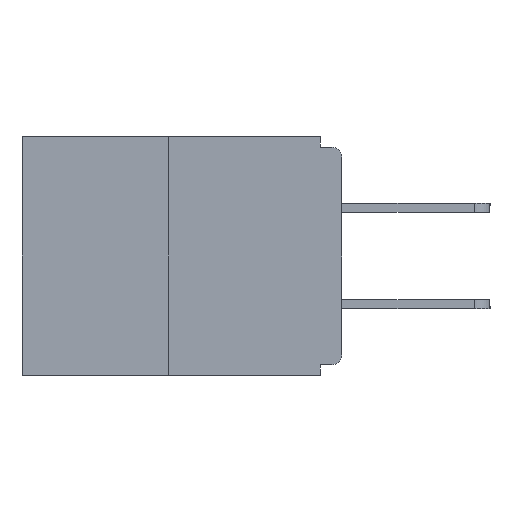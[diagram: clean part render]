
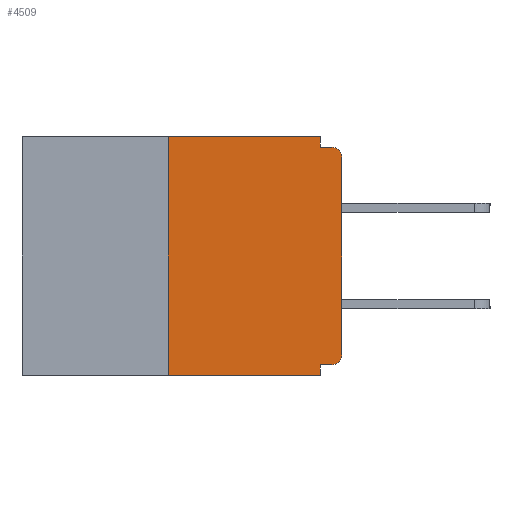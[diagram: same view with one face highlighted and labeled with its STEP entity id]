
A CAD part, left-side view. The second image highlights one B-rep face of the part: STEP entity #4509.
In plain terms, the highlighted planar face has unit normal (-1, 0, 0).
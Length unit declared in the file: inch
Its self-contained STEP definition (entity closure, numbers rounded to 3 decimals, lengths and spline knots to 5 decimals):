
#17 = DIRECTION ( 'NONE',  ( 0., 0., 1. ) ) ;
#65 = VECTOR ( 'NONE', #12326, 39.37008 ) ;
#394 = EDGE_CURVE ( 'NONE', #13748, #21394, #15729, .T. ) ;
#430 = VERTEX_POINT ( 'NONE', #3647 ) ;
#510 = VERTEX_POINT ( 'NONE', #16942 ) ;
#1112 = VECTOR ( 'NONE', #11327, 39.37008 ) ;
#1169 = EDGE_CURVE ( 'NONE', #23631, #23949, #14227, .T. ) ;
#2263 = DIRECTION ( 'NONE',  ( -1., 0., 0. ) ) ;
#2493 = CARTESIAN_POINT ( 'NONE',  ( 0., 0.031, 0. ) ) ;
#2647 = CARTESIAN_POINT ( 'NONE',  ( 0., 0.46, -0.343 ) ) ;
#2707 = DIRECTION ( 'NONE',  ( 0., 0., 1. ) ) ;
#2801 = DIRECTION ( 'NONE',  ( 0., 1., 0. ) ) ;
#2949 = ORIENTED_EDGE ( 'NONE', *, *, #7492, .F. ) ;
#3462 = LINE ( 'NONE', #6589, #19483 ) ;
#3647 = CARTESIAN_POINT ( 'NONE',  ( 0., 0.031, -0.328 ) ) ;
#3692 = CARTESIAN_POINT ( 'NONE',  ( 0., 0.46, 0. ) ) ;
#3781 = DIRECTION ( 'NONE',  ( 0., 0., -1. ) ) ;
#3813 = CARTESIAN_POINT ( 'NONE',  ( 0., 0.031, -0.015 ) ) ;
#4336 = CARTESIAN_POINT ( 'NONE',  ( 0., 0.25, -0.343 ) ) ;
#4509 = ADVANCED_FACE ( 'NONE', ( #15419 ), #11255, .F. ) ;
#4637 = ORIENTED_EDGE ( 'NONE', *, *, #15008, .T. ) ;
#4896 = DIRECTION ( 'NONE',  ( 0., 0., -1. ) ) ;
#5035 = CARTESIAN_POINT ( 'NONE',  ( 0., 0., -0.015 ) ) ;
#5761 = VECTOR ( 'NONE', #17707, 39.37008 ) ;
#5794 = CARTESIAN_POINT ( 'NONE',  ( 0., 0.031, -0.343 ) ) ;
#6016 = ORIENTED_EDGE ( 'NONE', *, *, #6807, .F. ) ;
#6589 = CARTESIAN_POINT ( 'NONE',  ( 0., 0., -0.328 ) ) ;
#6690 = VERTEX_POINT ( 'NONE', #3813 ) ;
#6807 = EDGE_CURVE ( 'NONE', #23949, #6690, #24477, .T. ) ;
#6901 = CARTESIAN_POINT ( 'NONE',  ( 0., 0.015, -0.313 ) ) ;
#6910 = LINE ( 'NONE', #2647, #65 ) ;
#7216 = LINE ( 'NONE', #5794, #10164 ) ;
#7260 = ORIENTED_EDGE ( 'NONE', *, *, #24002, .F. ) ;
#7492 = EDGE_CURVE ( 'NONE', #430, #23935, #7216, .T. ) ;
#8080 = CARTESIAN_POINT ( 'NONE',  ( 0., 0.031, -0.343 ) ) ;
#8311 = CARTESIAN_POINT ( 'NONE',  ( 0., 0.031, 0. ) ) ;
#8497 = VECTOR ( 'NONE', #10668, 39.37008 ) ;
#9319 = CARTESIAN_POINT ( 'NONE',  ( 0., 0., 0. ) ) ;
#9580 = CARTESIAN_POINT ( 'NONE',  ( 0., 0.46, 0. ) ) ;
#9623 = CARTESIAN_POINT ( 'NONE',  ( 0., 0.015, -0.015 ) ) ;
#9791 = EDGE_CURVE ( 'NONE', #19447, #23935, #6910, .T. ) ;
#10164 = VECTOR ( 'NONE', #3781, 39.37008 ) ;
#10453 = CARTESIAN_POINT ( 'NONE',  ( 0., 0., -0.313 ) ) ;
#10668 = DIRECTION ( 'NONE',  ( 0., -1., 0. ) ) ;
#10769 = CARTESIAN_POINT ( 'NONE',  ( 0., 0.015, -0.328 ) ) ;
#10823 = ORIENTED_EDGE ( 'NONE', *, *, #21679, .F. ) ;
#11255 = PLANE ( 'NONE',  #13940 ) ;
#11327 = DIRECTION ( 'NONE',  ( 0., -1., 0. ) ) ;
#11560 = ORIENTED_EDGE ( 'NONE', *, *, #14972, .T. ) ;
#12210 = EDGE_LOOP ( 'NONE', ( #12917, #7260, #21166, #2949, #17452, #22731, #11560, #4637, #10823, #6016 ) ) ;
#12326 = DIRECTION ( 'NONE',  ( 0., -1., 0. ) ) ;
#12917 = ORIENTED_EDGE ( 'NONE', *, *, #1169, .F. ) ;
#13135 = LINE ( 'NONE', #9319, #20820 ) ;
#13145 = EDGE_CURVE ( 'NONE', #13748, #430, #3462, .T. ) ;
#13678 = CARTESIAN_POINT ( 'NONE',  ( 0., 0.015, -0.03 ) ) ;
#13748 = VERTEX_POINT ( 'NONE', #10769 ) ;
#13940 = AXIS2_PLACEMENT_3D ( 'NONE', #3692, #20980, #16992 ) ;
#14227 = LINE ( 'NONE', #9580, #1112 ) ;
#14285 = CARTESIAN_POINT ( 'NONE',  ( 0., 0.25, 0. ) ) ;
#14972 = EDGE_CURVE ( 'NONE', #21394, #510, #13135, .T. ) ;
#15008 = EDGE_CURVE ( 'NONE', #510, #20783, #22622, .T. ) ;
#15419 = FACE_OUTER_BOUND ( 'NONE', #12210, .T. ) ;
#15729 = CIRCLE ( 'NONE', #16386, 0.015 ) ;
#16386 = AXIS2_PLACEMENT_3D ( 'NONE', #6901, #18250, #4896 ) ;
#16942 = CARTESIAN_POINT ( 'NONE',  ( 0., 0., -0.03 ) ) ;
#16992 = DIRECTION ( 'NONE',  ( 0., 0., -1. ) ) ;
#17411 = LINE ( 'NONE', #5035, #8497 ) ;
#17452 = ORIENTED_EDGE ( 'NONE', *, *, #13145, .F. ) ;
#17707 = DIRECTION ( 'NONE',  ( 0., 0., -1. ) ) ;
#18250 = DIRECTION ( 'NONE',  ( -1., 0., 0. ) ) ;
#18756 = VECTOR ( 'NONE', #2707, 39.37008 ) ;
#19447 = VERTEX_POINT ( 'NONE', #4336 ) ;
#19483 = VECTOR ( 'NONE', #2801, 39.37008 ) ;
#20783 = VERTEX_POINT ( 'NONE', #9623 ) ;
#20820 = VECTOR ( 'NONE', #17, 39.37008 ) ;
#20980 = DIRECTION ( 'NONE',  ( 1., 0., 0. ) ) ;
#21166 = ORIENTED_EDGE ( 'NONE', *, *, #9791, .T. ) ;
#21394 = VERTEX_POINT ( 'NONE', #10453 ) ;
#21679 = EDGE_CURVE ( 'NONE', #6690, #20783, #17411, .T. ) ;
#22612 = AXIS2_PLACEMENT_3D ( 'NONE', #13678, #2263, #23221 ) ;
#22622 = CIRCLE ( 'NONE', #22612, 0.015 ) ;
#22731 = ORIENTED_EDGE ( 'NONE', *, *, #394, .T. ) ;
#22786 = CARTESIAN_POINT ( 'NONE',  ( 0., 0.25, 0. ) ) ;
#23221 = DIRECTION ( 'NONE',  ( 0., 0., -1. ) ) ;
#23631 = VERTEX_POINT ( 'NONE', #22786 ) ;
#23815 = LINE ( 'NONE', #14285, #18756 ) ;
#23935 = VERTEX_POINT ( 'NONE', #8080 ) ;
#23949 = VERTEX_POINT ( 'NONE', #8311 ) ;
#24002 = EDGE_CURVE ( 'NONE', #19447, #23631, #23815, .T. ) ;
#24477 = LINE ( 'NONE', #2493, #5761 ) ;
